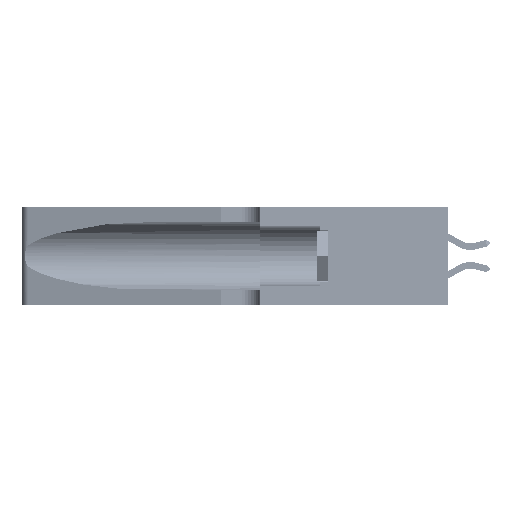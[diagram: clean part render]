
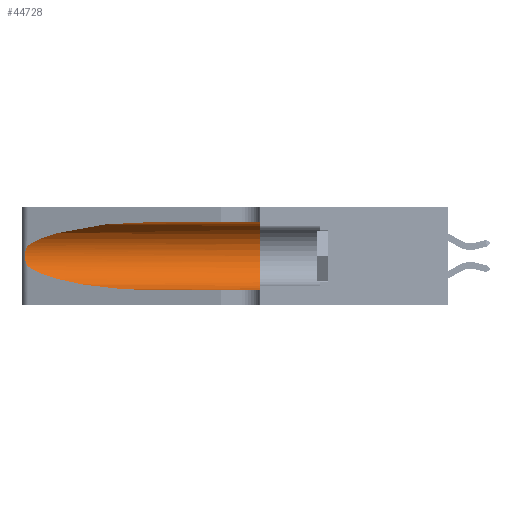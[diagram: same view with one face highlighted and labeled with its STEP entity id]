
A CAD part, left-side view. The second image highlights one B-rep face of the part: STEP entity #44728.
In plain terms, the highlighted cylindrical face has radius 3.308 mm (diameter 6.617 mm), a partial arc.
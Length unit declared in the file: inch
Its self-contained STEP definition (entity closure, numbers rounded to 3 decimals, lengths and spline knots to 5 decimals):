
#1565 = CARTESIAN_POINT ( 'NONE',  ( 0.25555, 1.22994, 0.2215 ) ) ;
#1753 = VERTEX_POINT ( 'NONE', #13613 ) ;
#1885 = CARTESIAN_POINT ( 'NONE',  ( 0.1305, 0.35, 0.185 ) ) ;
#1947 = VERTEX_POINT ( 'NONE', #32759 ) ;
#2384 = CARTESIAN_POINT ( 'NONE',  ( 0.25639, 1.23184, 0.21858 ) ) ;
#2718 =( BOUNDED_CURVE ( )  B_SPLINE_CURVE ( 3, ( #10591, #36733, #21555, #2861 ),
 .UNSPECIFIED., .F., .F. ) 
 B_SPLINE_CURVE_WITH_KNOTS ( ( 4, 4 ),
 ( 3.44316, 4.71239 ),
 .UNSPECIFIED. ) 
 CURVE ( )  GEOMETRIC_REPRESENTATION_ITEM ( )  RATIONAL_B_SPLINE_CURVE ( ( 1., 0.87, 0.87, 1. ) ) 
 REPRESENTATION_ITEM ( '' )  );
#2861 = CARTESIAN_POINT ( 'NONE',  ( 0.1305, 0.72297, 0.05475 ) ) ;
#3644 = VECTOR ( 'NONE', #39791, 39.37008 ) ;
#4000 = CARTESIAN_POINT ( 'NONE',  ( 0.25789, 1.23486, 0.15765 ) ) ;
#6148 = DIRECTION ( 'NONE',  ( 0., -1., 0. ) ) ;
#6471 = DIRECTION ( 'NONE',  ( 0., 0., -1. ) ) ;
#6820 = CYLINDRICAL_SURFACE ( 'NONE', #15228, 0.13025 ) ;
#6914 = EDGE_CURVE ( 'NONE', #13132, #15546, #20174, .T. ) ;
#7173 = CARTESIAN_POINT ( 'NONE',  ( 0.26018, 1.23835, 0.19895 ) ) ;
#8130 = EDGE_CURVE ( 'NONE', #15546, #1753, #21375, .T. ) ;
#9980 = CARTESIAN_POINT ( 'NONE',  ( 0.25787, 1.23484, 0.2124 ) ) ;
#10046 = ORIENTED_EDGE ( 'NONE', *, *, #37825, .T. ) ;
#10591 = CARTESIAN_POINT ( 'NONE',  ( 0.25487, 1.22718, 0.14631 ) ) ;
#12070 = CARTESIAN_POINT ( 'NONE',  ( 0.25555, 1.22993, 0.14849 ) ) ;
#12466 = CARTESIAN_POINT ( 'NONE',  ( 0.1305, 1.61858, 0.05475 ) ) ;
#13132 = VERTEX_POINT ( 'NONE', #20566 ) ;
#13613 = CARTESIAN_POINT ( 'NONE',  ( 0.25487, 1.22718, 0.14631 ) ) ;
#15228 = AXIS2_PLACEMENT_3D ( 'NONE', #24658, #6148, #6471 ) ;
#15546 = VERTEX_POINT ( 'NONE', #48393 ) ;
#16552 = CARTESIAN_POINT ( 'NONE',  ( 0.25487, 1.22718, 0.22369 ) ) ;
#18812 = CARTESIAN_POINT ( 'NONE',  ( 0.25856, 1.23593, 0.16098 ) ) ;
#19835 = EDGE_CURVE ( 'NONE', #1753, #1947, #2718, .T. ) ;
#20174 =( BOUNDED_CURVE ( )  B_SPLINE_CURVE ( 3, ( #36319, #32435, #29008, #25374 ),
 .UNSPECIFIED., .F., .F. ) 
 B_SPLINE_CURVE_WITH_KNOTS ( ( 4, 4 ),
 ( 1.5708, 2.84003 ),
 .UNSPECIFIED. ) 
 CURVE ( )  GEOMETRIC_REPRESENTATION_ITEM ( )  RATIONAL_B_SPLINE_CURVE ( ( 1., 0.87, 0.87, 1. ) ) 
 REPRESENTATION_ITEM ( '' )  );
#20566 = CARTESIAN_POINT ( 'NONE',  ( 0.1305, 0.72297, 0.31525 ) ) ;
#21181 = VERTEX_POINT ( 'NONE', #29790 ) ;
#21375 = B_SPLINE_CURVE_WITH_KNOTS ( 'NONE', 3,
 ( #16552, #1565, #2384, #9980, #44593, #7173, #37062, #26277, #44760, #18812, #4000, #41467, #12070, #45249 ),
 .UNSPECIFIED., .F., .F.,
 ( 4, 2, 2, 2, 2, 2, 4 ),
 ( 0., 0.00027, 0.00053, 0.00107, 0.0016, 0.00187, 0.00214 ),
 .UNSPECIFIED. ) ;
#21392 = LINE ( 'NONE', #12466, #28441 ) ;
#21555 = CARTESIAN_POINT ( 'NONE',  ( 0.18966, 0.96281, 0.05475 ) ) ;
#22640 = FACE_OUTER_BOUND ( 'NONE', #23814, .T. ) ;
#23814 = EDGE_LOOP ( 'NONE', ( #28883, #36228, #28744, #10046, #38489, #37852 ) ) ;
#24293 = CARTESIAN_POINT ( 'NONE',  ( 0.1305, 1.61858, 0.31525 ) ) ;
#24658 = CARTESIAN_POINT ( 'NONE',  ( 0.1305, 1.61858, 0.185 ) ) ;
#25374 = CARTESIAN_POINT ( 'NONE',  ( 0.25487, 1.22718, 0.22369 ) ) ;
#26273 = CIRCLE ( 'NONE', #33318, 0.13025 ) ;
#26277 = CARTESIAN_POINT ( 'NONE',  ( 0.26075, 1.23896, 0.178 ) ) ;
#28137 = DIRECTION ( 'NONE',  ( 0., 0., 1. ) ) ;
#28441 = VECTOR ( 'NONE', #38608, 39.37008 ) ;
#28744 = ORIENTED_EDGE ( 'NONE', *, *, #19835, .T. ) ;
#28883 = ORIENTED_EDGE ( 'NONE', *, *, #6914, .T. ) ;
#29008 = CARTESIAN_POINT ( 'NONE',  ( 0.2373, 1.15595, 0.28018 ) ) ;
#29790 = CARTESIAN_POINT ( 'NONE',  ( 0.1305, 0.35, 0.05475 ) ) ;
#30033 = LINE ( 'NONE', #24293, #3644 ) ;
#32435 = CARTESIAN_POINT ( 'NONE',  ( 0.18966, 0.96281, 0.31525 ) ) ;
#32664 = VERTEX_POINT ( 'NONE', #42203 ) ;
#32759 = CARTESIAN_POINT ( 'NONE',  ( 0.1305, 0.72297, 0.05475 ) ) ;
#33318 = AXIS2_PLACEMENT_3D ( 'NONE', #1885, #35148, #28137 ) ;
#35148 = DIRECTION ( 'NONE',  ( 0., 1., 0. ) ) ;
#36228 = ORIENTED_EDGE ( 'NONE', *, *, #8130, .T. ) ;
#36319 = CARTESIAN_POINT ( 'NONE',  ( 0.1305, 0.72297, 0.31525 ) ) ;
#36733 = CARTESIAN_POINT ( 'NONE',  ( 0.2373, 1.15595, 0.08982 ) ) ;
#37062 = CARTESIAN_POINT ( 'NONE',  ( 0.26075, 1.23896, 0.19203 ) ) ;
#37825 = EDGE_CURVE ( 'NONE', #1947, #21181, #21392, .T. ) ;
#37852 = ORIENTED_EDGE ( 'NONE', *, *, #39325, .F. ) ;
#38489 = ORIENTED_EDGE ( 'NONE', *, *, #42609, .F. ) ;
#38608 = DIRECTION ( 'NONE',  ( 0., -1., 0. ) ) ;
#39325 = EDGE_CURVE ( 'NONE', #13132, #32664, #30033, .T. ) ;
#39791 = DIRECTION ( 'NONE',  ( 0., -1., 0. ) ) ;
#41467 = CARTESIAN_POINT ( 'NONE',  ( 0.25639, 1.23186, 0.15144 ) ) ;
#42203 = CARTESIAN_POINT ( 'NONE',  ( 0.1305, 0.35, 0.31525 ) ) ;
#42609 = EDGE_CURVE ( 'NONE', #32664, #21181, #26273, .T. ) ;
#44593 = CARTESIAN_POINT ( 'NONE',  ( 0.25854, 1.2359, 0.20912 ) ) ;
#44728 = ADVANCED_FACE ( 'NONE', ( #22640 ), #6820, .F. ) ;
#44760 = CARTESIAN_POINT ( 'NONE',  ( 0.26017, 1.23833, 0.17102 ) ) ;
#45249 = CARTESIAN_POINT ( 'NONE',  ( 0.25487, 1.22718, 0.14631 ) ) ;
#48393 = CARTESIAN_POINT ( 'NONE',  ( 0.25487, 1.22718, 0.22369 ) ) ;
